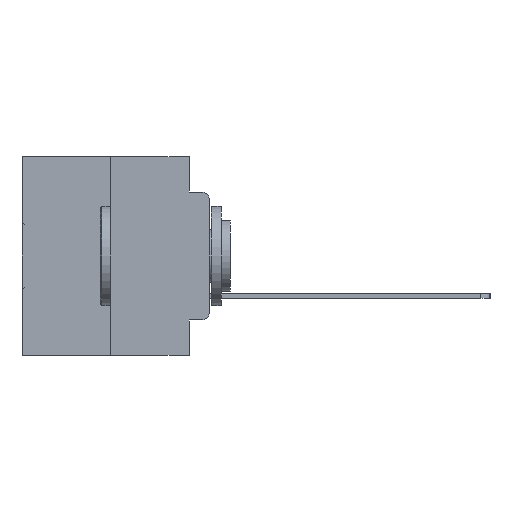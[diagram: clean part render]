
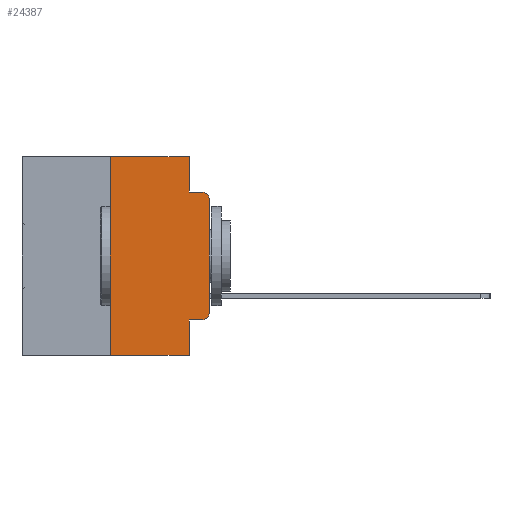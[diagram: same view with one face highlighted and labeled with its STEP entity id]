
A CAD part, left-side view. The second image highlights one B-rep face of the part: STEP entity #24387.
In plain terms, the highlighted planar face has unit normal (-1, 0, 0).
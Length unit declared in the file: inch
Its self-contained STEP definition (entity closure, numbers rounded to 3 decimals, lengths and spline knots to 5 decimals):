
#265 = DIRECTION ( 'NONE',  ( 1., 0., 0. ) ) ;
#498 = VERTEX_POINT ( 'NONE', #23548 ) ;
#1418 = ORIENTED_EDGE ( 'NONE', *, *, #28344, .T. ) ;
#1514 = LINE ( 'NONE', #27700, #27363 ) ;
#1671 = LINE ( 'NONE', #18480, #20937 ) ;
#2822 = EDGE_CURVE ( 'NONE', #12891, #20428, #16881, .T. ) ;
#2849 = DIRECTION ( 'NONE',  ( -1., 0., 0. ) ) ;
#3723 = ORIENTED_EDGE ( 'NONE', *, *, #21361, .T. ) ;
#4113 = AXIS2_PLACEMENT_3D ( 'NONE', #30263, #265, #17878 ) ;
#4312 = VECTOR ( 'NONE', #21264, 39.37008 ) ;
#4665 = CARTESIAN_POINT ( 'NONE',  ( 0., 0.051, -0.0885 ) ) ;
#5309 = CARTESIAN_POINT ( 'NONE',  ( 0., 0.473, -0.5 ) ) ;
#6203 = EDGE_CURVE ( 'NONE', #20428, #18960, #1514, .T. ) ;
#6266 = CARTESIAN_POINT ( 'NONE',  ( 0., 0.25, -0.5 ) ) ;
#6882 = CARTESIAN_POINT ( 'NONE',  ( 0., 0.02, -0.1085 ) ) ;
#6923 = VECTOR ( 'NONE', #27506, 39.37008 ) ;
#7513 = CARTESIAN_POINT ( 'NONE',  ( 0., 0.051, 0. ) ) ;
#7629 = CIRCLE ( 'NONE', #8808, 0.02 ) ;
#7860 = DIRECTION ( 'NONE',  ( 0., -1., 0. ) ) ;
#8808 = AXIS2_PLACEMENT_3D ( 'NONE', #6882, #24357, #9412 ) ;
#9202 = CARTESIAN_POINT ( 'NONE',  ( 0., 0.051, 0. ) ) ;
#9412 = DIRECTION ( 'NONE',  ( 0., 0., -1. ) ) ;
#10320 = VECTOR ( 'NONE', #19700, 39.37008 ) ;
#11515 = EDGE_LOOP ( 'NONE', ( #3723, #19104, #13986, #21431, #12043, #27647, #22602, #16758, #32307, #1418 ) ) ;
#12043 = ORIENTED_EDGE ( 'NONE', *, *, #6203, .F. ) ;
#12840 = PLANE ( 'NONE',  #4113 ) ;
#12891 = VERTEX_POINT ( 'NONE', #6266 ) ;
#13603 = EDGE_CURVE ( 'NONE', #18960, #23399, #25647, .T. ) ;
#13891 = EDGE_CURVE ( 'NONE', #12891, #15482, #16300, .T. ) ;
#13986 = ORIENTED_EDGE ( 'NONE', *, *, #31152, .F. ) ;
#15482 = VERTEX_POINT ( 'NONE', #20681 ) ;
#15983 = VERTEX_POINT ( 'NONE', #30090 ) ;
#16181 = LINE ( 'NONE', #4665, #10320 ) ;
#16300 = LINE ( 'NONE', #5309, #28760 ) ;
#16758 = ORIENTED_EDGE ( 'NONE', *, *, #30253, .F. ) ;
#16881 = LINE ( 'NONE', #31141, #4312 ) ;
#17878 = DIRECTION ( 'NONE',  ( 0., 0., -1. ) ) ;
#17899 = CARTESIAN_POINT ( 'NONE',  ( 0., 0.02, -0.3915 ) ) ;
#18279 = CIRCLE ( 'NONE', #28916, 0.02 ) ;
#18480 = CARTESIAN_POINT ( 'NONE',  ( 0., 0., 0. ) ) ;
#18960 = VERTEX_POINT ( 'NONE', #7513 ) ;
#19079 = VECTOR ( 'NONE', #24141, 39.37008 ) ;
#19104 = ORIENTED_EDGE ( 'NONE', *, *, #20949, .T. ) ;
#19700 = DIRECTION ( 'NONE',  ( 0., -1., 0. ) ) ;
#20414 = DIRECTION ( 'NONE',  ( 0., 0., -1. ) ) ;
#20428 = VERTEX_POINT ( 'NONE', #23920 ) ;
#20551 = VERTEX_POINT ( 'NONE', #24337 ) ;
#20681 = CARTESIAN_POINT ( 'NONE',  ( 0., 0.051, -0.5 ) ) ;
#20937 = VECTOR ( 'NONE', #25939, 39.37008 ) ;
#20949 = EDGE_CURVE ( 'NONE', #21221, #15983, #7629, .T. ) ;
#21221 = VERTEX_POINT ( 'NONE', #27935 ) ;
#21264 = DIRECTION ( 'NONE',  ( 0., 0., 1. ) ) ;
#21333 = VECTOR ( 'NONE', #25482, 39.37008 ) ;
#21361 = EDGE_CURVE ( 'NONE', #20551, #21221, #1671, .T. ) ;
#21431 = ORIENTED_EDGE ( 'NONE', *, *, #13603, .F. ) ;
#22602 = ORIENTED_EDGE ( 'NONE', *, *, #13891, .T. ) ;
#22810 = DIRECTION ( 'NONE',  ( 0., -1., 0. ) ) ;
#23000 = CARTESIAN_POINT ( 'NONE',  ( 0., 0.051, 0. ) ) ;
#23399 = VERTEX_POINT ( 'NONE', #24540 ) ;
#23548 = CARTESIAN_POINT ( 'NONE',  ( 0., 0.02, -0.4115 ) ) ;
#23920 = CARTESIAN_POINT ( 'NONE',  ( 0., 0.25, 0. ) ) ;
#24141 = DIRECTION ( 'NONE',  ( 0., 0., -1. ) ) ;
#24200 = CARTESIAN_POINT ( 'NONE',  ( 0., 0.051, -0.4115 ) ) ;
#24337 = CARTESIAN_POINT ( 'NONE',  ( 0., 0., -0.3915 ) ) ;
#24357 = DIRECTION ( 'NONE',  ( -1., 0., 0. ) ) ;
#24387 = ADVANCED_FACE ( 'NONE', ( #30176 ), #12840, .F. ) ;
#24540 = CARTESIAN_POINT ( 'NONE',  ( 0., 0.051, -0.0885 ) ) ;
#25001 = CARTESIAN_POINT ( 'NONE',  ( 0., 0.051, -0.4115 ) ) ;
#25482 = DIRECTION ( 'NONE',  ( 0., 0., -1. ) ) ;
#25647 = LINE ( 'NONE', #9202, #19079 ) ;
#25939 = DIRECTION ( 'NONE',  ( 0., 0., 1. ) ) ;
#26854 = LINE ( 'NONE', #25001, #6923 ) ;
#27096 = EDGE_CURVE ( 'NONE', #29968, #498, #26854, .T. ) ;
#27363 = VECTOR ( 'NONE', #22810, 39.37008 ) ;
#27506 = DIRECTION ( 'NONE',  ( 0., -1., 0. ) ) ;
#27647 = ORIENTED_EDGE ( 'NONE', *, *, #2822, .F. ) ;
#27700 = CARTESIAN_POINT ( 'NONE',  ( 0., 0.473, 0. ) ) ;
#27921 = LINE ( 'NONE', #23000, #21333 ) ;
#27935 = CARTESIAN_POINT ( 'NONE',  ( 0., 0., -0.1085 ) ) ;
#28344 = EDGE_CURVE ( 'NONE', #498, #20551, #18279, .T. ) ;
#28760 = VECTOR ( 'NONE', #7860, 39.37008 ) ;
#28916 = AXIS2_PLACEMENT_3D ( 'NONE', #17899, #2849, #20414 ) ;
#29968 = VERTEX_POINT ( 'NONE', #24200 ) ;
#30090 = CARTESIAN_POINT ( 'NONE',  ( 0., 0.02, -0.0885 ) ) ;
#30176 = FACE_OUTER_BOUND ( 'NONE', #11515, .T. ) ;
#30253 = EDGE_CURVE ( 'NONE', #29968, #15482, #27921, .T. ) ;
#30263 = CARTESIAN_POINT ( 'NONE',  ( 0., 0.473, 0. ) ) ;
#31141 = CARTESIAN_POINT ( 'NONE',  ( 0., 0.25, 0. ) ) ;
#31152 = EDGE_CURVE ( 'NONE', #23399, #15983, #16181, .T. ) ;
#32307 = ORIENTED_EDGE ( 'NONE', *, *, #27096, .T. ) ;
